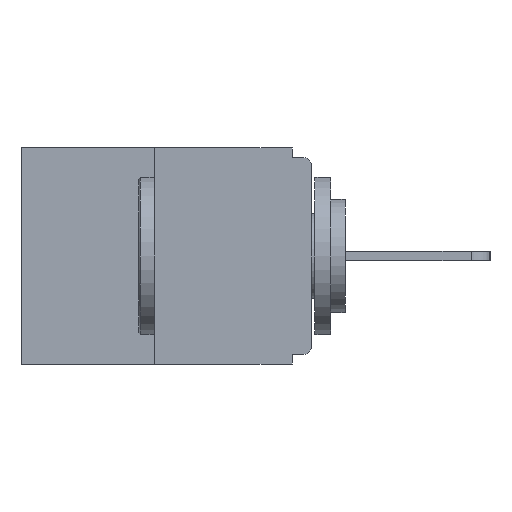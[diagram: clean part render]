
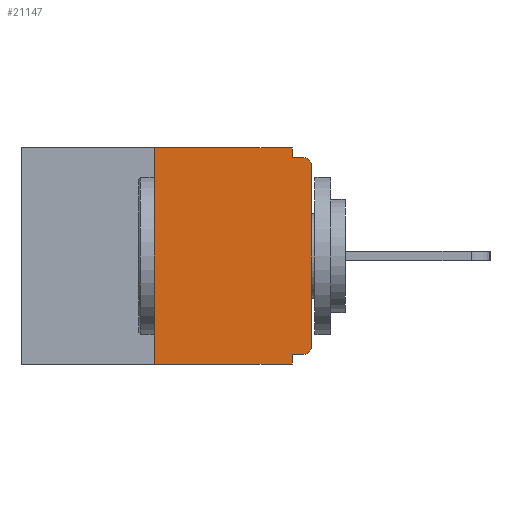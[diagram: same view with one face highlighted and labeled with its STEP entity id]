
A CAD part, left-side view. The second image highlights one B-rep face of the part: STEP entity #21147.
In plain terms, the highlighted planar face has unit normal (-1, 0, 0).
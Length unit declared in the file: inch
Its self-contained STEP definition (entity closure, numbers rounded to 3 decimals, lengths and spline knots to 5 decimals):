
#141 = CARTESIAN_POINT ( 'NONE',  ( 0., 0.015, -0.313 ) ) ;
#175 = DIRECTION ( 'NONE',  ( -1., 0., 0. ) ) ;
#525 = DIRECTION ( 'NONE',  ( 0., -1., 0. ) ) ;
#620 = EDGE_CURVE ( 'NONE', #10181, #14990, #19496, .T. ) ;
#637 = LINE ( 'NONE', #2465, #10078 ) ;
#692 = EDGE_CURVE ( 'NONE', #3166, #25167, #23461, .T. ) ;
#1038 = VERTEX_POINT ( 'NONE', #13850 ) ;
#1071 = EDGE_CURVE ( 'NONE', #1038, #11396, #14078, .T. ) ;
#1304 = ORIENTED_EDGE ( 'NONE', *, *, #14537, .F. ) ;
#1627 = CARTESIAN_POINT ( 'NONE',  ( 0., 0., -0.015 ) ) ;
#1929 = FACE_OUTER_BOUND ( 'NONE', #6108, .T. ) ;
#1947 = DIRECTION ( 'NONE',  ( 0., 0., -1. ) ) ;
#2079 = EDGE_CURVE ( 'NONE', #21456, #25167, #3358, .T. ) ;
#2465 = CARTESIAN_POINT ( 'NONE',  ( 0., 0., 0. ) ) ;
#2783 = DIRECTION ( 'NONE',  ( 0., 0., 1. ) ) ;
#3166 = VERTEX_POINT ( 'NONE', #19948 ) ;
#3173 = ORIENTED_EDGE ( 'NONE', *, *, #620, .F. ) ;
#3358 = LINE ( 'NONE', #7928, #23993 ) ;
#4488 = ORIENTED_EDGE ( 'NONE', *, *, #22707, .F. ) ;
#4705 = DIRECTION ( 'NONE',  ( 0., 0., -1. ) ) ;
#5423 = ORIENTED_EDGE ( 'NONE', *, *, #692, .F. ) ;
#5913 = CARTESIAN_POINT ( 'NONE',  ( 0., 0., -0.328 ) ) ;
#6108 = EDGE_LOOP ( 'NONE', ( #3173, #24433, #14493, #5423, #1304, #7303, #23829, #19249, #25056, #4488 ) ) ;
#6111 = EDGE_CURVE ( 'NONE', #21456, #10181, #18277, .T. ) ;
#6145 = CARTESIAN_POINT ( 'NONE',  ( 0., 0.46, 0. ) ) ;
#6454 = EDGE_CURVE ( 'NONE', #25095, #13932, #25329, .T. ) ;
#7303 = ORIENTED_EDGE ( 'NONE', *, *, #1071, .T. ) ;
#7458 = CARTESIAN_POINT ( 'NONE',  ( 0., 0.031, -0.015 ) ) ;
#7518 = LINE ( 'NONE', #14700, #17568 ) ;
#7596 = CARTESIAN_POINT ( 'NONE',  ( 0., 0.031, -0.343 ) ) ;
#7600 = VECTOR ( 'NONE', #2783, 39.37008 ) ;
#7928 = CARTESIAN_POINT ( 'NONE',  ( 0., 0.46, -0.343 ) ) ;
#8179 = DIRECTION ( 'NONE',  ( 1., 0., 0. ) ) ;
#8438 = DIRECTION ( 'NONE',  ( 0., 0., 1. ) ) ;
#9413 = CARTESIAN_POINT ( 'NONE',  ( 0., 0., -0.313 ) ) ;
#9429 = VECTOR ( 'NONE', #525, 39.37008 ) ;
#9556 = CARTESIAN_POINT ( 'NONE',  ( 0., 0.25, 0. ) ) ;
#10078 = VECTOR ( 'NONE', #8438, 39.37008 ) ;
#10181 = VERTEX_POINT ( 'NONE', #9556 ) ;
#10360 = CARTESIAN_POINT ( 'NONE',  ( 0., 0.46, 0. ) ) ;
#10549 = CARTESIAN_POINT ( 'NONE',  ( 0., 0.015, -0.03 ) ) ;
#11117 = DIRECTION ( 'NONE',  ( 0., -1., 0. ) ) ;
#11396 = VERTEX_POINT ( 'NONE', #9413 ) ;
#12128 = PLANE ( 'NONE',  #13764 ) ;
#12604 = DIRECTION ( 'NONE',  ( 0., 0., -1. ) ) ;
#13259 = CARTESIAN_POINT ( 'NONE',  ( 0., 0.031, 0. ) ) ;
#13496 = VECTOR ( 'NONE', #11117, 39.37008 ) ;
#13704 = LINE ( 'NONE', #5913, #17804 ) ;
#13764 = AXIS2_PLACEMENT_3D ( 'NONE', #6145, #8179, #22177 ) ;
#13850 = CARTESIAN_POINT ( 'NONE',  ( 0., 0.015, -0.328 ) ) ;
#13932 = VERTEX_POINT ( 'NONE', #23909 ) ;
#14078 = CIRCLE ( 'NONE', #17487, 0.015 ) ;
#14200 = VERTEX_POINT ( 'NONE', #18913 ) ;
#14493 = ORIENTED_EDGE ( 'NONE', *, *, #2079, .T. ) ;
#14537 = EDGE_CURVE ( 'NONE', #1038, #3166, #13704, .T. ) ;
#14640 = CIRCLE ( 'NONE', #17225, 0.015 ) ;
#14700 = CARTESIAN_POINT ( 'NONE',  ( 0., 0.031, 0. ) ) ;
#14990 = VERTEX_POINT ( 'NONE', #13259 ) ;
#15034 = DIRECTION ( 'NONE',  ( 0., 0., -1. ) ) ;
#16977 = VECTOR ( 'NONE', #15034, 39.37008 ) ;
#17225 = AXIS2_PLACEMENT_3D ( 'NONE', #10549, #24499, #12604 ) ;
#17487 = AXIS2_PLACEMENT_3D ( 'NONE', #141, #175, #1947 ) ;
#17568 = VECTOR ( 'NONE', #4705, 39.37008 ) ;
#17703 = DIRECTION ( 'NONE',  ( 0., -1., 0. ) ) ;
#17804 = VECTOR ( 'NONE', #25769, 39.37008 ) ;
#18144 = CARTESIAN_POINT ( 'NONE',  ( 0., 0.25, 0. ) ) ;
#18277 = LINE ( 'NONE', #18144, #7600 ) ;
#18913 = CARTESIAN_POINT ( 'NONE',  ( 0., 0., -0.03 ) ) ;
#19249 = ORIENTED_EDGE ( 'NONE', *, *, #24335, .T. ) ;
#19496 = LINE ( 'NONE', #10360, #13496 ) ;
#19651 = CARTESIAN_POINT ( 'NONE',  ( 0., 0.031, -0.343 ) ) ;
#19948 = CARTESIAN_POINT ( 'NONE',  ( 0., 0.031, -0.328 ) ) ;
#21115 = CARTESIAN_POINT ( 'NONE',  ( 0., 0.25, -0.343 ) ) ;
#21147 = ADVANCED_FACE ( 'NONE', ( #1929 ), #12128, .F. ) ;
#21242 = EDGE_CURVE ( 'NONE', #11396, #14200, #637, .T. ) ;
#21456 = VERTEX_POINT ( 'NONE', #21115 ) ;
#22177 = DIRECTION ( 'NONE',  ( 0., 0., -1. ) ) ;
#22707 = EDGE_CURVE ( 'NONE', #14990, #25095, #7518, .T. ) ;
#23461 = LINE ( 'NONE', #7596, #16977 ) ;
#23829 = ORIENTED_EDGE ( 'NONE', *, *, #21242, .T. ) ;
#23909 = CARTESIAN_POINT ( 'NONE',  ( 0., 0.015, -0.015 ) ) ;
#23993 = VECTOR ( 'NONE', #17703, 39.37008 ) ;
#24335 = EDGE_CURVE ( 'NONE', #14200, #13932, #14640, .T. ) ;
#24433 = ORIENTED_EDGE ( 'NONE', *, *, #6111, .F. ) ;
#24499 = DIRECTION ( 'NONE',  ( -1., 0., 0. ) ) ;
#25056 = ORIENTED_EDGE ( 'NONE', *, *, #6454, .F. ) ;
#25095 = VERTEX_POINT ( 'NONE', #7458 ) ;
#25167 = VERTEX_POINT ( 'NONE', #19651 ) ;
#25329 = LINE ( 'NONE', #1627, #9429 ) ;
#25769 = DIRECTION ( 'NONE',  ( 0., 1., 0. ) ) ;
